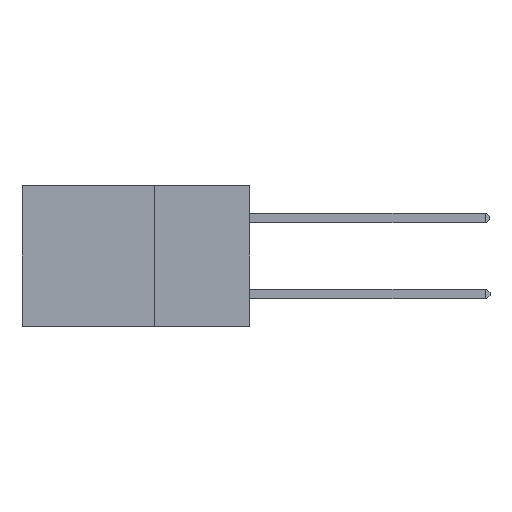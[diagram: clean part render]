
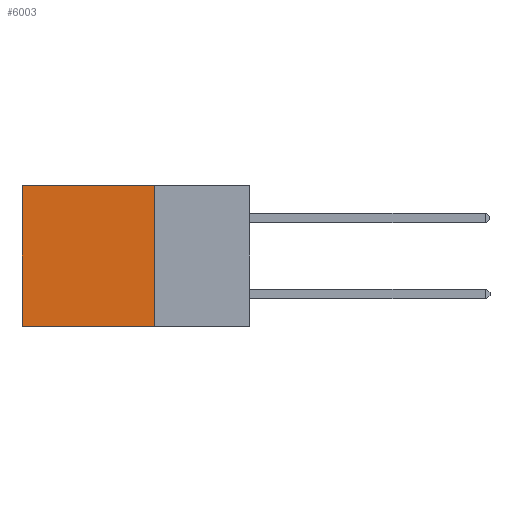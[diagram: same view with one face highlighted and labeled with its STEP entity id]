
A CAD part, left-side view. The second image highlights one B-rep face of the part: STEP entity #6003.
In plain terms, the highlighted planar face has unit normal (-1, 0, 0).
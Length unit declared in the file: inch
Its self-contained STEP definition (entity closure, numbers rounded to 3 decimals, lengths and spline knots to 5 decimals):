
#2744 = CARTESIAN_POINT ( 'NONE',  ( 0.2875, 0.6, 0. ) ) ;
#2819 = ORIENTED_EDGE ( 'NONE', *, *, #9933, .F. ) ;
#3921 = CARTESIAN_POINT ( 'NONE',  ( 0.2875, 0.25, -0.37 ) ) ;
#3932 = CARTESIAN_POINT ( 'NONE',  ( 0.2875, 0.25, 0. ) ) ;
#4235 = LINE ( 'NONE', #14033, #17308 ) ;
#5540 = EDGE_CURVE ( 'NONE', #22143, #13716, #10673, .T. ) ;
#5699 = DIRECTION ( 'NONE',  ( 0., 0., -1. ) ) ;
#6003 = ADVANCED_FACE ( 'NONE', ( #14869 ), #10994, .F. ) ;
#8682 = DIRECTION ( 'NONE',  ( 0., 1., 0. ) ) ;
#9751 = DIRECTION ( 'NONE',  ( 0., 0., -1. ) ) ;
#9933 = EDGE_CURVE ( 'NONE', #13716, #21588, #20646, .T. ) ;
#10291 = DIRECTION ( 'NONE',  ( 0., 0., -1. ) ) ;
#10673 = LINE ( 'NONE', #22130, #20092 ) ;
#10797 = EDGE_CURVE ( 'NONE', #22143, #12102, #4235, .T. ) ;
#10994 = PLANE ( 'NONE',  #21702 ) ;
#11240 = VECTOR ( 'NONE', #13106, 39.37008 ) ;
#12102 = VERTEX_POINT ( 'NONE', #2744 ) ;
#13106 = DIRECTION ( 'NONE',  ( 0., 1., 0. ) ) ;
#13246 = VECTOR ( 'NONE', #10291, 39.37008 ) ;
#13716 = VERTEX_POINT ( 'NONE', #3921 ) ;
#14033 = CARTESIAN_POINT ( 'NONE',  ( 0.2875, 0.25, 0. ) ) ;
#14869 = FACE_OUTER_BOUND ( 'NONE', #15394, .T. ) ;
#15087 = ORIENTED_EDGE ( 'NONE', *, *, #10797, .T. ) ;
#15394 = EDGE_LOOP ( 'NONE', ( #22903, #2819, #19624, #15087 ) ) ;
#15457 = CARTESIAN_POINT ( 'NONE',  ( 0.2875, 0.25, 0. ) ) ;
#16377 = DIRECTION ( 'NONE',  ( 1., 0., 0. ) ) ;
#17308 = VECTOR ( 'NONE', #8682, 39.37008 ) ;
#17389 = CARTESIAN_POINT ( 'NONE',  ( 0.2875, 0.6, 0. ) ) ;
#17494 = CARTESIAN_POINT ( 'NONE',  ( 0.2875, 0.6, -0.37 ) ) ;
#18500 = LINE ( 'NONE', #17389, #13246 ) ;
#19624 = ORIENTED_EDGE ( 'NONE', *, *, #5540, .F. ) ;
#20092 = VECTOR ( 'NONE', #9751, 39.37008 ) ;
#20646 = LINE ( 'NONE', #21880, #11240 ) ;
#21588 = VERTEX_POINT ( 'NONE', #17494 ) ;
#21702 = AXIS2_PLACEMENT_3D ( 'NONE', #3932, #16377, #5699 ) ;
#21880 = CARTESIAN_POINT ( 'NONE',  ( 0.2875, 0.25, -0.37 ) ) ;
#22130 = CARTESIAN_POINT ( 'NONE',  ( 0.2875, 0.25, 0. ) ) ;
#22143 = VERTEX_POINT ( 'NONE', #15457 ) ;
#22203 = EDGE_CURVE ( 'NONE', #12102, #21588, #18500, .T. ) ;
#22903 = ORIENTED_EDGE ( 'NONE', *, *, #22203, .T. ) ;
